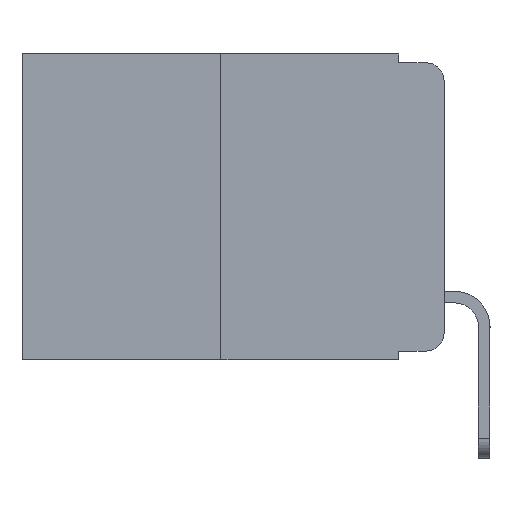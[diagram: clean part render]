
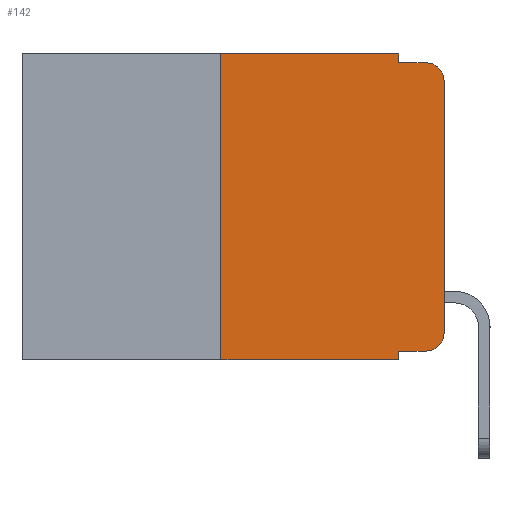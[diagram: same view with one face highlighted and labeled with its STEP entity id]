
A CAD part, left-side view. The second image highlights one B-rep face of the part: STEP entity #142.
In plain terms, the highlighted planar face has unit normal (-1, 0, 0).
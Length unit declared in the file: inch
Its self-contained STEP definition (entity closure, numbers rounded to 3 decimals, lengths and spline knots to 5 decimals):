
#26 = DIRECTION ( 'NONE',  ( 0., 0., -1. ) ) ;
#142 = ADVANCED_FACE ( 'NONE', ( #2455 ), #13703, .F. ) ;
#195 = CARTESIAN_POINT ( 'NONE',  ( 0., 0.02, -0.333 ) ) ;
#244 = DIRECTION ( 'NONE',  ( 0., -1., 0. ) ) ;
#959 = CARTESIAN_POINT ( 'NONE',  ( 0., 0.02, -0.01 ) ) ;
#964 = CARTESIAN_POINT ( 'NONE',  ( 0., 0.25, 0. ) ) ;
#1268 = DIRECTION ( 'NONE',  ( 0., 0., -1. ) ) ;
#1420 = CARTESIAN_POINT ( 'NONE',  ( 0., 0.02, -0.313 ) ) ;
#1440 = LINE ( 'NONE', #5063, #12535 ) ;
#1650 = VERTEX_POINT ( 'NONE', #3170 ) ;
#1849 = ORIENTED_EDGE ( 'NONE', *, *, #3386, .T. ) ;
#1911 = ORIENTED_EDGE ( 'NONE', *, *, #4440, .F. ) ;
#1937 = CARTESIAN_POINT ( 'NONE',  ( 0., 0.051, -0.01 ) ) ;
#2119 = LINE ( 'NONE', #3180, #5070 ) ;
#2123 = LINE ( 'NONE', #964, #14878 ) ;
#2455 = FACE_OUTER_BOUND ( 'NONE', #7528, .T. ) ;
#2482 = CARTESIAN_POINT ( 'NONE',  ( 0., 0.25, 0. ) ) ;
#2622 = ORIENTED_EDGE ( 'NONE', *, *, #8246, .T. ) ;
#2777 = EDGE_CURVE ( 'NONE', #6289, #4808, #3925, .T. ) ;
#3170 = CARTESIAN_POINT ( 'NONE',  ( 0., 0.051, -0.01 ) ) ;
#3180 = CARTESIAN_POINT ( 'NONE',  ( 0., 0.051, 0. ) ) ;
#3386 = EDGE_CURVE ( 'NONE', #6289, #12759, #5388, .T. ) ;
#3515 = CARTESIAN_POINT ( 'NONE',  ( 0., 0.02, -0.03 ) ) ;
#3540 = DIRECTION ( 'NONE',  ( 0., 0., -1. ) ) ;
#3542 = AXIS2_PLACEMENT_3D ( 'NONE', #1420, #14191, #7924 ) ;
#3710 = VERTEX_POINT ( 'NONE', #3963 ) ;
#3777 = DIRECTION ( 'NONE',  ( 1., 0., 0. ) ) ;
#3820 = EDGE_CURVE ( 'NONE', #12759, #11014, #5903, .T. ) ;
#3889 = EDGE_CURVE ( 'NONE', #14792, #14503, #2123, .T. ) ;
#3925 = LINE ( 'NONE', #5159, #7212 ) ;
#3963 = CARTESIAN_POINT ( 'NONE',  ( 0., 0., -0.03 ) ) ;
#4293 = LINE ( 'NONE', #10489, #14046 ) ;
#4440 = EDGE_CURVE ( 'NONE', #14503, #16243, #1440, .T. ) ;
#4502 = ORIENTED_EDGE ( 'NONE', *, *, #3820, .T. ) ;
#4808 = VERTEX_POINT ( 'NONE', #13319 ) ;
#5063 = CARTESIAN_POINT ( 'NONE',  ( 0., 0.473, 0. ) ) ;
#5070 = VECTOR ( 'NONE', #12185, 39.37008 ) ;
#5078 = CARTESIAN_POINT ( 'NONE',  ( 0., 0.25, -0.343 ) ) ;
#5159 = CARTESIAN_POINT ( 'NONE',  ( 0., 0.051, 0. ) ) ;
#5388 = LINE ( 'NONE', #6545, #12249 ) ;
#5482 = AXIS2_PLACEMENT_3D ( 'NONE', #3515, #8546, #1268 ) ;
#5903 = CIRCLE ( 'NONE', #3542, 0.02 ) ;
#6094 = ORIENTED_EDGE ( 'NONE', *, *, #2777, .F. ) ;
#6289 = VERTEX_POINT ( 'NONE', #11661 ) ;
#6298 = EDGE_CURVE ( 'NONE', #14792, #4808, #4293, .T. ) ;
#6466 = DIRECTION ( 'NONE',  ( 0., -1., 0. ) ) ;
#6545 = CARTESIAN_POINT ( 'NONE',  ( 0., 0.051, -0.333 ) ) ;
#6953 = EDGE_CURVE ( 'NONE', #1650, #11364, #9448, .T. ) ;
#6964 = DIRECTION ( 'NONE',  ( 0., -1., 0. ) ) ;
#7212 = VECTOR ( 'NONE', #26, 39.37008 ) ;
#7485 = ORIENTED_EDGE ( 'NONE', *, *, #6298, .T. ) ;
#7528 = EDGE_LOOP ( 'NONE', ( #12352, #2622, #10513, #15963, #1911, #15293, #7485, #6094, #1849, #4502 ) ) ;
#7924 = DIRECTION ( 'NONE',  ( 0., 0., -1. ) ) ;
#7933 = DIRECTION ( 'NONE',  ( 0., -1., 0. ) ) ;
#8099 = CIRCLE ( 'NONE', #5482, 0.02 ) ;
#8128 = VECTOR ( 'NONE', #6964, 39.37008 ) ;
#8246 = EDGE_CURVE ( 'NONE', #3710, #11364, #8099, .T. ) ;
#8451 = CARTESIAN_POINT ( 'NONE',  ( 0., 0., 0. ) ) ;
#8546 = DIRECTION ( 'NONE',  ( -1., 0., 0. ) ) ;
#9448 = LINE ( 'NONE', #1937, #8128 ) ;
#9880 = EDGE_CURVE ( 'NONE', #11014, #3710, #10919, .T. ) ;
#10489 = CARTESIAN_POINT ( 'NONE',  ( 0., 0.473, -0.343 ) ) ;
#10513 = ORIENTED_EDGE ( 'NONE', *, *, #6953, .F. ) ;
#10919 = LINE ( 'NONE', #8451, #14182 ) ;
#11014 = VERTEX_POINT ( 'NONE', #15492 ) ;
#11120 = DIRECTION ( 'NONE',  ( 0., 0., 1. ) ) ;
#11159 = EDGE_CURVE ( 'NONE', #16243, #1650, #2119, .T. ) ;
#11364 = VERTEX_POINT ( 'NONE', #959 ) ;
#11661 = CARTESIAN_POINT ( 'NONE',  ( 0., 0.051, -0.333 ) ) ;
#12088 = DIRECTION ( 'NONE',  ( 0., 0., 1. ) ) ;
#12185 = DIRECTION ( 'NONE',  ( 0., 0., -1. ) ) ;
#12249 = VECTOR ( 'NONE', #244, 39.37008 ) ;
#12352 = ORIENTED_EDGE ( 'NONE', *, *, #9880, .T. ) ;
#12535 = VECTOR ( 'NONE', #6466, 39.37008 ) ;
#12619 = CARTESIAN_POINT ( 'NONE',  ( 0., 0.473, 0. ) ) ;
#12759 = VERTEX_POINT ( 'NONE', #195 ) ;
#13319 = CARTESIAN_POINT ( 'NONE',  ( 0., 0.051, -0.343 ) ) ;
#13703 = PLANE ( 'NONE',  #15277 ) ;
#14046 = VECTOR ( 'NONE', #7933, 39.37008 ) ;
#14182 = VECTOR ( 'NONE', #12088, 39.37008 ) ;
#14191 = DIRECTION ( 'NONE',  ( -1., 0., 0. ) ) ;
#14482 = CARTESIAN_POINT ( 'NONE',  ( 0., 0.051, 0. ) ) ;
#14503 = VERTEX_POINT ( 'NONE', #2482 ) ;
#14792 = VERTEX_POINT ( 'NONE', #5078 ) ;
#14878 = VECTOR ( 'NONE', #11120, 39.37008 ) ;
#15277 = AXIS2_PLACEMENT_3D ( 'NONE', #12619, #3777, #3540 ) ;
#15293 = ORIENTED_EDGE ( 'NONE', *, *, #3889, .F. ) ;
#15492 = CARTESIAN_POINT ( 'NONE',  ( 0., 0., -0.313 ) ) ;
#15963 = ORIENTED_EDGE ( 'NONE', *, *, #11159, .F. ) ;
#16243 = VERTEX_POINT ( 'NONE', #14482 ) ;
